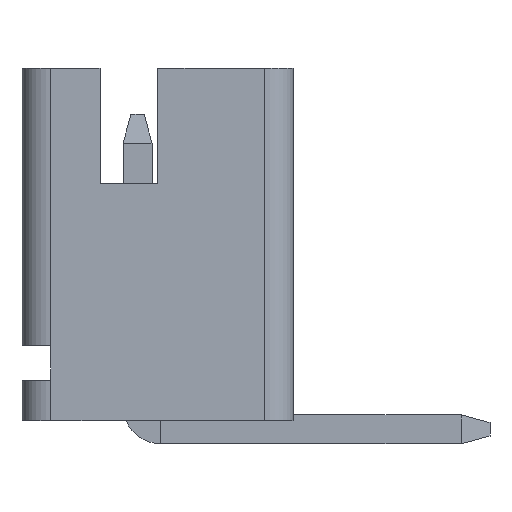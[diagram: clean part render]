
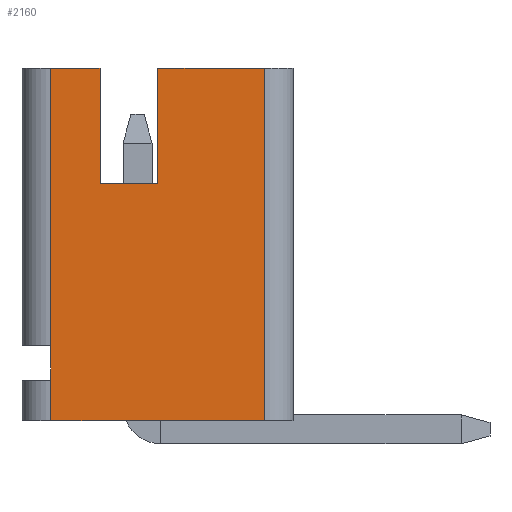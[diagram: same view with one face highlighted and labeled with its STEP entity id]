
A CAD part, left-side view. The second image highlights one B-rep face of the part: STEP entity #2160.
In plain terms, the highlighted planar face has unit normal (-1, 0, 0).
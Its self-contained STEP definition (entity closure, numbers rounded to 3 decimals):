
#35 = LINE ( 'NONE', #674, #2332 ) ;
#51 = DIRECTION ( 'NONE',  ( 0., 0., -1. ) ) ;
#61 = LINE ( 'NONE', #2953, #174 ) ;
#88 = ORIENTED_EDGE ( 'NONE', *, *, #1282, .T. ) ;
#154 = VERTEX_POINT ( 'NONE', #3976 ) ;
#171 = VECTOR ( 'NONE', #51, 1000. ) ;
#174 = VECTOR ( 'NONE', #979, 1000. ) ;
#339 = LINE ( 'NONE', #639, #2703 ) ;
#432 = VECTOR ( 'NONE', #3962, 1000. ) ;
#534 = ORIENTED_EDGE ( 'NONE', *, *, #2067, .T. ) ;
#573 = AXIS2_PLACEMENT_3D ( 'NONE', #2450, #1417, #1763 ) ;
#591 = ORIENTED_EDGE ( 'NONE', *, *, #3390, .T. ) ;
#639 = CARTESIAN_POINT ( 'NONE',  ( -2., 0.65, 4.1 ) ) ;
#649 = VECTOR ( 'NONE', #4046, 1000. ) ;
#674 = CARTESIAN_POINT ( 'NONE',  ( -2., -2.2, 0. ) ) ;
#676 = VERTEX_POINT ( 'NONE', #3675 ) ;
#683 = EDGE_CURVE ( 'NONE', #881, #2245, #2665, .T. ) ;
#745 = CARTESIAN_POINT ( 'NONE',  ( -2., 2., 6.1 ) ) ;
#813 = VERTEX_POINT ( 'NONE', #3161 ) ;
#815 = ORIENTED_EDGE ( 'NONE', *, *, #1609, .T. ) ;
#881 = VERTEX_POINT ( 'NONE', #2171 ) ;
#956 = VECTOR ( 'NONE', #2827, 1000. ) ;
#979 = DIRECTION ( 'NONE',  ( 0., 0., -1. ) ) ;
#995 = DIRECTION ( 'NONE',  ( 0., 1., 0. ) ) ;
#1035 = CARTESIAN_POINT ( 'NONE',  ( -2., -0.35, 6.1 ) ) ;
#1069 = DIRECTION ( 'NONE',  ( 0., 1., 0. ) ) ;
#1083 = DIRECTION ( 'NONE',  ( 0., 0., 1. ) ) ;
#1134 = CARTESIAN_POINT ( 'NONE',  ( -2., 1.5, 1.3 ) ) ;
#1282 = EDGE_CURVE ( 'NONE', #2903, #676, #1820, .T. ) ;
#1315 = CARTESIAN_POINT ( 'NONE',  ( -2., 1.5, 0. ) ) ;
#1328 = VECTOR ( 'NONE', #1725, 1000. ) ;
#1330 = VERTEX_POINT ( 'NONE', #4092 ) ;
#1396 = EDGE_LOOP ( 'NONE', ( #534, #3144, #815, #4213, #3523, #591, #1960, #3367, #88, #3372 ) ) ;
#1417 = DIRECTION ( 'NONE',  ( -1., 0., 0. ) ) ;
#1429 = CARTESIAN_POINT ( 'NONE',  ( -2., 0.65, 6.1 ) ) ;
#1502 = VERTEX_POINT ( 'NONE', #1917 ) ;
#1609 = EDGE_CURVE ( 'NONE', #1502, #881, #2667, .T. ) ;
#1619 = EDGE_CURVE ( 'NONE', #3156, #1502, #35, .T. ) ;
#1633 = LINE ( 'NONE', #2662, #432 ) ;
#1688 = CARTESIAN_POINT ( 'NONE',  ( -2., 1.5, 1.3 ) ) ;
#1725 = DIRECTION ( 'NONE',  ( 0., 0., -1. ) ) ;
#1763 = DIRECTION ( 'NONE',  ( 0., -1., 0. ) ) ;
#1820 = LINE ( 'NONE', #1134, #956 ) ;
#1906 = CARTESIAN_POINT ( 'NONE',  ( -2., 1.5, 0. ) ) ;
#1917 = CARTESIAN_POINT ( 'NONE',  ( -2., -2.2, 6.1 ) ) ;
#1947 = DIRECTION ( 'NONE',  ( 0., 1., 0. ) ) ;
#1960 = ORIENTED_EDGE ( 'NONE', *, *, #3279, .T. ) ;
#1962 = LINE ( 'NONE', #1315, #1328 ) ;
#2056 = CARTESIAN_POINT ( 'NONE',  ( -2., -0.35, 6.1 ) ) ;
#2067 = EDGE_CURVE ( 'NONE', #2400, #3156, #1633, .T. ) ;
#2122 = FACE_OUTER_BOUND ( 'NONE', #1396, .T. ) ;
#2160 = ADVANCED_FACE ( 'NONE', ( #2122 ), #2469, .T. ) ;
#2171 = CARTESIAN_POINT ( 'NONE',  ( -2., -0.35, 6.1 ) ) ;
#2245 = VERTEX_POINT ( 'NONE', #2730 ) ;
#2332 = VECTOR ( 'NONE', #1083, 1000. ) ;
#2400 = VERTEX_POINT ( 'NONE', #1906 ) ;
#2435 = VECTOR ( 'NONE', #1069, 1000. ) ;
#2450 = CARTESIAN_POINT ( 'NONE',  ( -2., 0., 0. ) ) ;
#2468 = EDGE_CURVE ( 'NONE', #2245, #1330, #339, .T. ) ;
#2469 = PLANE ( 'NONE',  #573 ) ;
#2662 = CARTESIAN_POINT ( 'NONE',  ( -2., 2., 0. ) ) ;
#2665 = LINE ( 'NONE', #2056, #171 ) ;
#2667 = LINE ( 'NONE', #1035, #2755 ) ;
#2703 = VECTOR ( 'NONE', #1947, 1000. ) ;
#2730 = CARTESIAN_POINT ( 'NONE',  ( -2., -0.35, 4.1 ) ) ;
#2755 = VECTOR ( 'NONE', #995, 1000. ) ;
#2827 = DIRECTION ( 'NONE',  ( 0., 0., -1. ) ) ;
#2903 = VERTEX_POINT ( 'NONE', #1688 ) ;
#2953 = CARTESIAN_POINT ( 'NONE',  ( -2., 1.5, 0. ) ) ;
#2964 = EDGE_CURVE ( 'NONE', #154, #2903, #61, .T. ) ;
#3144 = ORIENTED_EDGE ( 'NONE', *, *, #1619, .T. ) ;
#3151 = LINE ( 'NONE', #1429, #649 ) ;
#3156 = VERTEX_POINT ( 'NONE', #3934 ) ;
#3161 = CARTESIAN_POINT ( 'NONE',  ( -2., 0.65, 6.1 ) ) ;
#3229 = EDGE_CURVE ( 'NONE', #676, #2400, #1962, .T. ) ;
#3279 = EDGE_CURVE ( 'NONE', #813, #154, #3323, .T. ) ;
#3323 = LINE ( 'NONE', #745, #2435 ) ;
#3367 = ORIENTED_EDGE ( 'NONE', *, *, #2964, .T. ) ;
#3372 = ORIENTED_EDGE ( 'NONE', *, *, #3229, .T. ) ;
#3390 = EDGE_CURVE ( 'NONE', #1330, #813, #3151, .T. ) ;
#3523 = ORIENTED_EDGE ( 'NONE', *, *, #2468, .T. ) ;
#3675 = CARTESIAN_POINT ( 'NONE',  ( -2., 1.5, 0.7 ) ) ;
#3934 = CARTESIAN_POINT ( 'NONE',  ( -2., -2.2, 0. ) ) ;
#3962 = DIRECTION ( 'NONE',  ( 0., -1., 0. ) ) ;
#3976 = CARTESIAN_POINT ( 'NONE',  ( -2., 1.5, 6.1 ) ) ;
#4046 = DIRECTION ( 'NONE',  ( 0., 0., 1. ) ) ;
#4092 = CARTESIAN_POINT ( 'NONE',  ( -2., 0.65, 4.1 ) ) ;
#4213 = ORIENTED_EDGE ( 'NONE', *, *, #683, .T. ) ;
